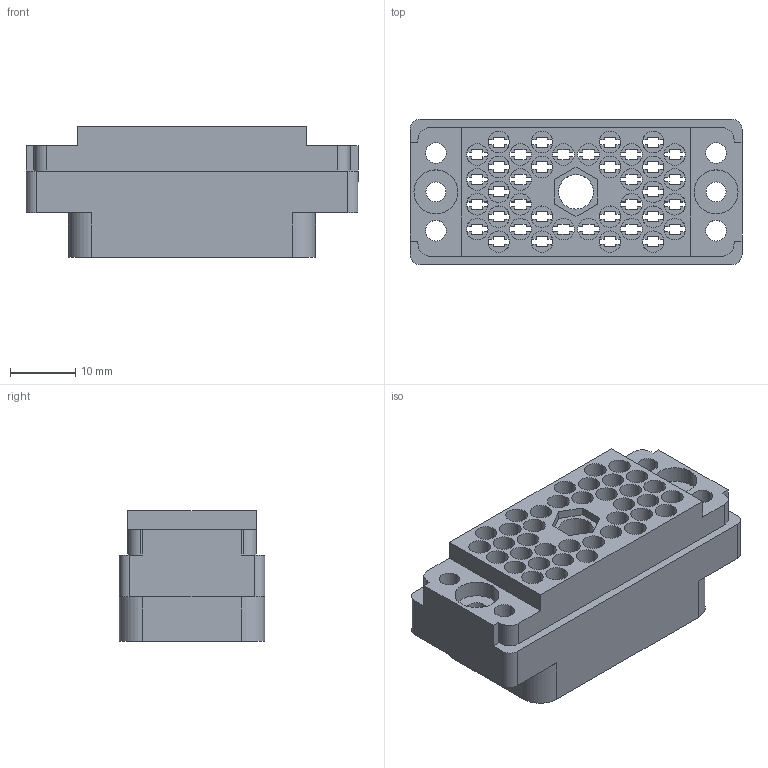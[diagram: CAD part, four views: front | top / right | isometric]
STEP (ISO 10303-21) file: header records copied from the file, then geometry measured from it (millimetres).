
FILE_DESCRIPTION (( 'STEP AP203' ), '1' );
FILE_NAME ('516-038-000-100.STEP', '2020-03-09T17:37:55', ( '' ), ( '' ), 'SwSTEP 2.0', 'SolidWorks 2016', '' );
FILE_SCHEMA (( 'CONFIG_CONTROL_DESIGN' ));
Length unit declared in the file: inch
Products named in the file (2): 516 Plug Insulator_038; 516-038-000-100
Assembly tree (1 placements, depth 2):
  516-038-000-100
    516 Plug Insulator_038
Bounding box: 50.8 x 22.25 x 20.04 mm (x, y, z)
Volume: 8636.7 mm3; surface area: 11468.7 mm2
Topology: 1 solids, 1 shells, 886 faces, 2600 edges, 1732 vertices
Faces by surface type: plane 641, cylinder 243, cone 2
Entity records: 29810 total; most frequent: CARTESIAN_POINT 5222, ORIENTED_EDGE 5200, DIRECTION 5018, EDGE_CURVE 2600, LINE 1962, VECTOR 1962, VERTEX_POINT 1732, AXIS2_PLACEMENT_3D 1528
